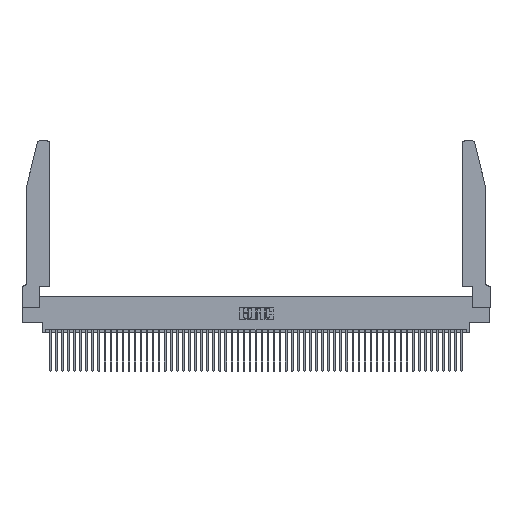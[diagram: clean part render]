
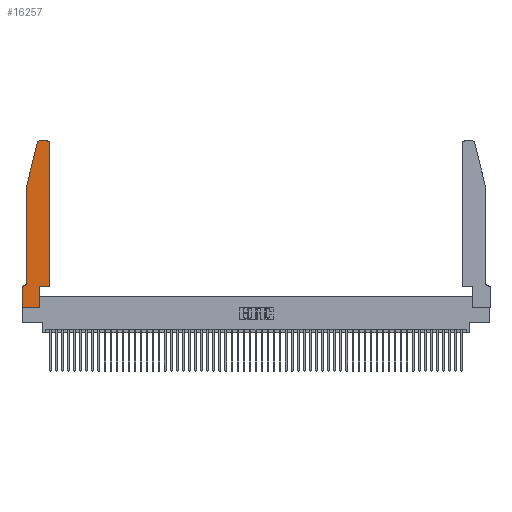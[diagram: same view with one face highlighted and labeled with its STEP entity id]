
A CAD part, top view. The second image highlights one B-rep face of the part: STEP entity #16257.
In plain terms, the highlighted planar face has unit normal (0, 0, 1).
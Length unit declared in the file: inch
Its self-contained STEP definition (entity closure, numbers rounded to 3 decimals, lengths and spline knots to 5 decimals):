
#141 = CARTESIAN_POINT ( 'NONE',  ( 0.0755, 0.42, 0.37 ) ) ;
#593 = CARTESIAN_POINT ( 'NONE',  ( 0.284, 2.72, 0.37 ) ) ;
#812 = EDGE_CURVE ( 'NONE', #52199, #43145, #29986, .T. ) ;
#1206 = VERTEX_POINT ( 'NONE', #36477 ) ;
#2460 = CARTESIAN_POINT ( 'NONE',  ( 0.0055, 0.35, 0.37 ) ) ;
#2547 = ORIENTED_EDGE ( 'NONE', *, *, #17652, .T. ) ;
#3550 = CARTESIAN_POINT ( 'NONE',  ( 0.4205, 2.75, 0.37 ) ) ;
#3920 = VERTEX_POINT ( 'NONE', #20212 ) ;
#4597 = VECTOR ( 'NONE', #28104, 39.37008 ) ;
#4964 = DIRECTION ( 'NONE',  ( 1., 0., 0. ) ) ;
#5019 = EDGE_CURVE ( 'NONE', #8960, #8248, #53463, .T. ) ;
#6126 = ORIENTED_EDGE ( 'NONE', *, *, #33734, .T. ) ;
#6193 = CIRCLE ( 'NONE', #21807, 0.07 ) ;
#7257 = LINE ( 'NONE', #23769, #4597 ) ;
#8233 = EDGE_CURVE ( 'NONE', #51390, #51658, #14442, .T. ) ;
#8248 = VERTEX_POINT ( 'NONE', #19486 ) ;
#8438 = VERTEX_POINT ( 'NONE', #37835 ) ;
#8584 = LINE ( 'NONE', #29331, #15933 ) ;
#8960 = VERTEX_POINT ( 'NONE', #37202 ) ;
#9674 = EDGE_CURVE ( 'NONE', #23396, #3920, #20322, .T. ) ;
#9742 = ORIENTED_EDGE ( 'NONE', *, *, #812, .T. ) ;
#10467 = AXIS2_PLACEMENT_3D ( 'NONE', #50877, #25367, #55141 ) ;
#10995 = CIRCLE ( 'NONE', #30587, 0.03 ) ;
#12020 = EDGE_LOOP ( 'NONE', ( #32993, #40314, #32270, #6126, #32452, #33749, #13165, #51480, #9742, #52212, #37020, #2547 ) ) ;
#12168 = DIRECTION ( 'NONE',  ( 0., -1., 0. ) ) ;
#12451 = EDGE_CURVE ( 'NONE', #43145, #1206, #8584, .T. ) ;
#12505 = CARTESIAN_POINT ( 'NONE',  ( 0.2865, 0.35, 0.37 ) ) ;
#12720 = CARTESIAN_POINT ( 'NONE',  ( 0.2865, 0.35, 0.37 ) ) ;
#13165 = ORIENTED_EDGE ( 'NONE', *, *, #35736, .T. ) ;
#13891 = CARTESIAN_POINT ( 'NONE',  ( 0.4505, 0.35, 0.37 ) ) ;
#14442 = LINE ( 'NONE', #14985, #37240 ) ;
#14925 = LINE ( 'NONE', #13891, #25012 ) ;
#14985 = CARTESIAN_POINT ( 'NONE',  ( 0.2605, 2.75, 0.37 ) ) ;
#15099 = DIRECTION ( 'NONE',  ( 0., 0., -1. ) ) ;
#15933 = VECTOR ( 'NONE', #50527, 39.37008 ) ;
#16257 = ADVANCED_FACE ( 'NONE', ( #35929 ), #20231, .T. ) ;
#17652 = EDGE_CURVE ( 'NONE', #8438, #51390, #24348, .T. ) ;
#17851 = EDGE_CURVE ( 'NONE', #1206, #8438, #14925, .T. ) ;
#19486 = CARTESIAN_POINT ( 'NONE',  ( 0.0755, 2., 0.37 ) ) ;
#19893 = DIRECTION ( 'NONE',  ( -0.239, -0.971, 0. ) ) ;
#20212 = CARTESIAN_POINT ( 'NONE',  ( 0., 0.35, 0.37 ) ) ;
#20231 = PLANE ( 'NONE',  #40560 ) ;
#20322 = LINE ( 'NONE', #23940, #30393 ) ;
#21807 = AXIS2_PLACEMENT_3D ( 'NONE', #40765, #15099, #45028 ) ;
#23396 = VERTEX_POINT ( 'NONE', #2460 ) ;
#23769 = CARTESIAN_POINT ( 'NONE',  ( 0., 0., 0.37 ) ) ;
#23940 = CARTESIAN_POINT ( 'NONE',  ( 0.0755, 0.35, 0.37 ) ) ;
#24348 = CIRCLE ( 'NONE', #10467, 0.03 ) ;
#24541 = DIRECTION ( 'NONE',  ( 1., 0., 0. ) ) ;
#25012 = VECTOR ( 'NONE', #43826, 39.37008 ) ;
#25367 = DIRECTION ( 'NONE',  ( 0., 0., 1. ) ) ;
#26337 = VERTEX_POINT ( 'NONE', #47933 ) ;
#27412 = EDGE_CURVE ( 'NONE', #51658, #8960, #10995, .T. ) ;
#28104 = DIRECTION ( 'NONE',  ( 1., 0., 0. ) ) ;
#28664 = CARTESIAN_POINT ( 'NONE',  ( 0., 0.35, 0.37 ) ) ;
#29105 = LINE ( 'NONE', #33746, #40468 ) ;
#29331 = CARTESIAN_POINT ( 'NONE',  ( 0.4505, 0.35, 0.37 ) ) ;
#29986 = LINE ( 'NONE', #12505, #52626 ) ;
#30393 = VECTOR ( 'NONE', #49509, 39.37008 ) ;
#30587 = AXIS2_PLACEMENT_3D ( 'NONE', #593, #30664, #4964 ) ;
#30664 = DIRECTION ( 'NONE',  ( 0., 0., 1. ) ) ;
#32270 = ORIENTED_EDGE ( 'NONE', *, *, #5019, .T. ) ;
#32452 = ORIENTED_EDGE ( 'NONE', *, *, #34211, .T. ) ;
#32993 = ORIENTED_EDGE ( 'NONE', *, *, #8233, .T. ) ;
#33734 = EDGE_CURVE ( 'NONE', #8248, #50956, #29105, .T. ) ;
#33746 = CARTESIAN_POINT ( 'NONE',  ( 0.0755, 2., 0.37 ) ) ;
#33749 = ORIENTED_EDGE ( 'NONE', *, *, #9674, .T. ) ;
#34211 = EDGE_CURVE ( 'NONE', #50956, #23396, #6193, .T. ) ;
#34321 = CARTESIAN_POINT ( 'NONE',  ( 0., 0., 0.37 ) ) ;
#34875 = VECTOR ( 'NONE', #46917, 39.37008 ) ;
#35736 = EDGE_CURVE ( 'NONE', #3920, #26337, #36211, .T. ) ;
#35929 = FACE_OUTER_BOUND ( 'NONE', #12020, .T. ) ;
#36211 = LINE ( 'NONE', #34321, #34875 ) ;
#36477 = CARTESIAN_POINT ( 'NONE',  ( 0.4505, 0.35, 0.37 ) ) ;
#36814 = EDGE_CURVE ( 'NONE', #26337, #52199, #7257, .T. ) ;
#37020 = ORIENTED_EDGE ( 'NONE', *, *, #17851, .T. ) ;
#37202 = CARTESIAN_POINT ( 'NONE',  ( 0.25487, 2.72718, 0.37 ) ) ;
#37240 = VECTOR ( 'NONE', #49188, 39.37008 ) ;
#37835 = CARTESIAN_POINT ( 'NONE',  ( 0.4505, 2.72, 0.37 ) ) ;
#40229 = CARTESIAN_POINT ( 'NONE',  ( 0.2865, 0., 0.37 ) ) ;
#40314 = ORIENTED_EDGE ( 'NONE', *, *, #27412, .T. ) ;
#40468 = VECTOR ( 'NONE', #12168, 39.37008 ) ;
#40560 = AXIS2_PLACEMENT_3D ( 'NONE', #28664, #50066, #24541 ) ;
#40765 = CARTESIAN_POINT ( 'NONE',  ( 0.0055, 0.42, 0.37 ) ) ;
#42193 = VECTOR ( 'NONE', #19893, 39.37008 ) ;
#42439 = DIRECTION ( 'NONE',  ( 0., 1., 0. ) ) ;
#43145 = VERTEX_POINT ( 'NONE', #12720 ) ;
#43816 = CARTESIAN_POINT ( 'NONE',  ( 0.284, 2.75, 0.37 ) ) ;
#43826 = DIRECTION ( 'NONE',  ( 0., 1., 0. ) ) ;
#45028 = DIRECTION ( 'NONE',  ( -1., 0., 0. ) ) ;
#46917 = DIRECTION ( 'NONE',  ( 0., -1., 0. ) ) ;
#47933 = CARTESIAN_POINT ( 'NONE',  ( 0., 0., 0.37 ) ) ;
#49188 = DIRECTION ( 'NONE',  ( -1., 0., 0. ) ) ;
#49509 = DIRECTION ( 'NONE',  ( -1., 0., 0. ) ) ;
#49759 = CARTESIAN_POINT ( 'NONE',  ( 0.0755, 2., 0.37 ) ) ;
#50066 = DIRECTION ( 'NONE',  ( 0., 0., 1. ) ) ;
#50527 = DIRECTION ( 'NONE',  ( 1., 0., 0. ) ) ;
#50877 = CARTESIAN_POINT ( 'NONE',  ( 0.4205, 2.72, 0.37 ) ) ;
#50956 = VERTEX_POINT ( 'NONE', #141 ) ;
#51390 = VERTEX_POINT ( 'NONE', #3550 ) ;
#51480 = ORIENTED_EDGE ( 'NONE', *, *, #36814, .T. ) ;
#51658 = VERTEX_POINT ( 'NONE', #43816 ) ;
#52199 = VERTEX_POINT ( 'NONE', #40229 ) ;
#52212 = ORIENTED_EDGE ( 'NONE', *, *, #12451, .T. ) ;
#52626 = VECTOR ( 'NONE', #42439, 39.37008 ) ;
#53463 = LINE ( 'NONE', #49759, #42193 ) ;
#55141 = DIRECTION ( 'NONE',  ( 1., 0., 0. ) ) ;
